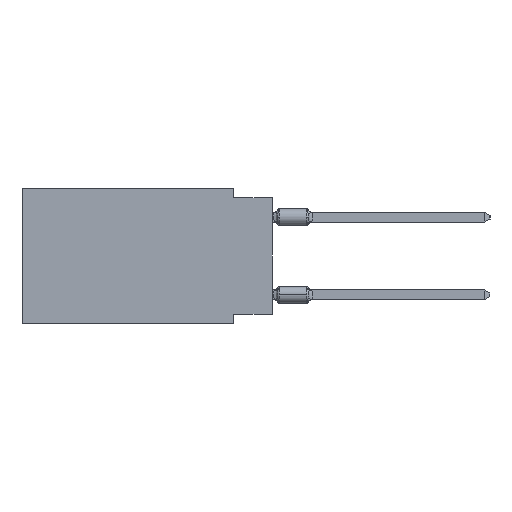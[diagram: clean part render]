
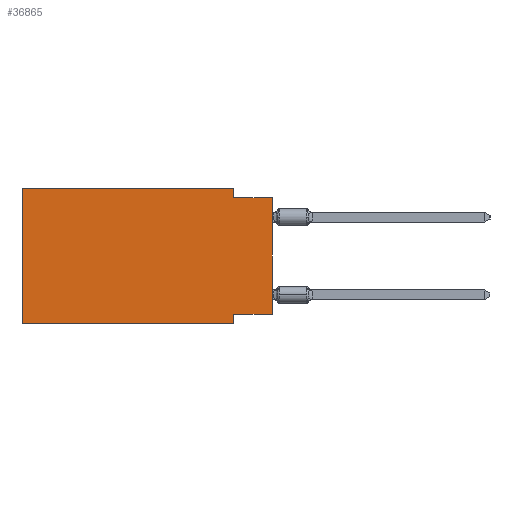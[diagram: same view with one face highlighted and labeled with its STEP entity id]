
A CAD part, left-side view. The second image highlights one B-rep face of the part: STEP entity #36865.
In plain terms, the highlighted planar face has unit normal (-1, 0, 0).
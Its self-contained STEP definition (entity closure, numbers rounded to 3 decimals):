
#1626 = DIRECTION ( 'NONE',  ( 0., 0., 1. ) ) ;
#1993 = EDGE_CURVE ( 'NONE', #29415, #22176, #4188, .T. ) ;
#2007 = VERTEX_POINT ( 'NONE', #15912 ) ;
#2010 = DIRECTION ( 'NONE',  ( 0., -1., 0. ) ) ;
#3365 = ORIENTED_EDGE ( 'NONE', *, *, #37098, .T. ) ;
#4188 = LINE ( 'NONE', #23028, #39161 ) ;
#6048 = VECTOR ( 'NONE', #14821, 1000. ) ;
#6485 = LINE ( 'NONE', #24861, #11275 ) ;
#7389 = VERTEX_POINT ( 'NONE', #19228 ) ;
#8598 = DIRECTION ( 'NONE',  ( 0., 0., -1. ) ) ;
#8862 = CARTESIAN_POINT ( 'NONE',  ( 0., 2.54, -8.89 ) ) ;
#9400 = PLANE ( 'NONE',  #43436 ) ;
#11106 = CARTESIAN_POINT ( 'NONE',  ( 0., 0., -0.635 ) ) ;
#11275 = VECTOR ( 'NONE', #1626, 1000. ) ;
#11316 = CARTESIAN_POINT ( 'NONE',  ( 0., 16.383, -8.89 ) ) ;
#12327 = ORIENTED_EDGE ( 'NONE', *, *, #23816, .F. ) ;
#12683 = ORIENTED_EDGE ( 'NONE', *, *, #23114, .F. ) ;
#13638 = ORIENTED_EDGE ( 'NONE', *, *, #15799, .F. ) ;
#13661 = DIRECTION ( 'NONE',  ( 0., 0., 1. ) ) ;
#13902 = ORIENTED_EDGE ( 'NONE', *, *, #27110, .T. ) ;
#14384 = VERTEX_POINT ( 'NONE', #41503 ) ;
#14821 = DIRECTION ( 'NONE',  ( 0., 1., 0. ) ) ;
#15799 = EDGE_CURVE ( 'NONE', #14384, #2007, #17329, .T. ) ;
#15912 = CARTESIAN_POINT ( 'NONE',  ( 0., 16.383, 0. ) ) ;
#16814 = CARTESIAN_POINT ( 'NONE',  ( 0., 2.54, -0.635 ) ) ;
#17329 = LINE ( 'NONE', #47178, #32038 ) ;
#17548 = VERTEX_POINT ( 'NONE', #16814 ) ;
#18170 = DIRECTION ( 'NONE',  ( 0., -1., 0. ) ) ;
#19228 = CARTESIAN_POINT ( 'NONE',  ( 0., 2.54, 0. ) ) ;
#20042 = VECTOR ( 'NONE', #47074, 1000. ) ;
#20574 = VECTOR ( 'NONE', #25578, 1000. ) ;
#20878 = VERTEX_POINT ( 'NONE', #27230 ) ;
#21083 = LINE ( 'NONE', #31626, #23262 ) ;
#21482 = ORIENTED_EDGE ( 'NONE', *, *, #42717, .F. ) ;
#22176 = VERTEX_POINT ( 'NONE', #8862 ) ;
#23028 = CARTESIAN_POINT ( 'NONE',  ( 0., 2.54, -8.89 ) ) ;
#23114 = EDGE_CURVE ( 'NONE', #17548, #47420, #32166, .T. ) ;
#23262 = VECTOR ( 'NONE', #2010, 1000. ) ;
#23543 = EDGE_CURVE ( 'NONE', #20878, #29415, #29516, .T. ) ;
#23816 = EDGE_CURVE ( 'NONE', #2007, #7389, #21083, .T. ) ;
#24861 = CARTESIAN_POINT ( 'NONE',  ( 0., 0., 0. ) ) ;
#25578 = DIRECTION ( 'NONE',  ( 0., 0., -1. ) ) ;
#26435 = CARTESIAN_POINT ( 'NONE',  ( 0., 2.54, -8.255 ) ) ;
#27110 = EDGE_CURVE ( 'NONE', #20878, #47420, #6485, .T. ) ;
#27230 = CARTESIAN_POINT ( 'NONE',  ( 0., 0., -8.255 ) ) ;
#27253 = ORIENTED_EDGE ( 'NONE', *, *, #1993, .F. ) ;
#29415 = VERTEX_POINT ( 'NONE', #26435 ) ;
#29516 = LINE ( 'NONE', #29761, #6048 ) ;
#29761 = CARTESIAN_POINT ( 'NONE',  ( 0., 0., -8.255 ) ) ;
#31626 = CARTESIAN_POINT ( 'NONE',  ( 0., 16.383, 0. ) ) ;
#32038 = VECTOR ( 'NONE', #13661, 1000. ) ;
#32166 = LINE ( 'NONE', #46850, #20042 ) ;
#32380 = FACE_OUTER_BOUND ( 'NONE', #34636, .T. ) ;
#34636 = EDGE_LOOP ( 'NONE', ( #13902, #12683, #21482, #12327, #13638, #3365, #27253, #37313 ) ) ;
#35892 = CARTESIAN_POINT ( 'NONE',  ( 0., 2.54, 0. ) ) ;
#36547 = LINE ( 'NONE', #11316, #42641 ) ;
#36598 = LINE ( 'NONE', #35892, #20574 ) ;
#36865 = ADVANCED_FACE ( 'NONE', ( #32380 ), #9400, .F. ) ;
#37098 = EDGE_CURVE ( 'NONE', #14384, #22176, #36547, .T. ) ;
#37313 = ORIENTED_EDGE ( 'NONE', *, *, #23543, .F. ) ;
#39161 = VECTOR ( 'NONE', #8598, 1000. ) ;
#41503 = CARTESIAN_POINT ( 'NONE',  ( 0., 16.383, -8.89 ) ) ;
#42641 = VECTOR ( 'NONE', #18170, 1000. ) ;
#42687 = CARTESIAN_POINT ( 'NONE',  ( 0., 16.383, 0. ) ) ;
#42717 = EDGE_CURVE ( 'NONE', #7389, #17548, #36598, .T. ) ;
#43393 = DIRECTION ( 'NONE',  ( 1., 0., 0. ) ) ;
#43436 = AXIS2_PLACEMENT_3D ( 'NONE', #42687, #43393, #46832 ) ;
#46832 = DIRECTION ( 'NONE',  ( 0., 0., -1. ) ) ;
#46850 = CARTESIAN_POINT ( 'NONE',  ( 0., 0., -0.635 ) ) ;
#47074 = DIRECTION ( 'NONE',  ( 0., -1., 0. ) ) ;
#47178 = CARTESIAN_POINT ( 'NONE',  ( 0., 16.383, 0. ) ) ;
#47420 = VERTEX_POINT ( 'NONE', #11106 ) ;
